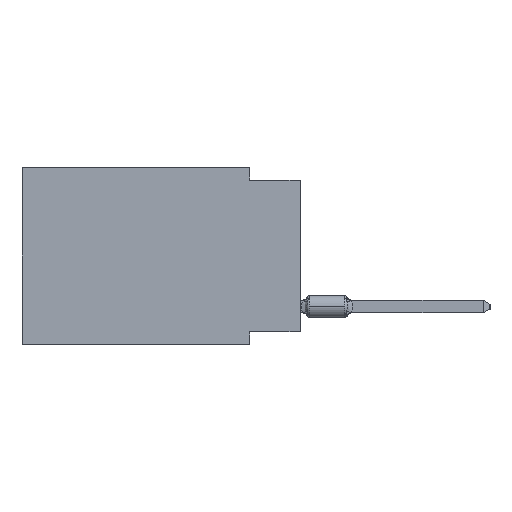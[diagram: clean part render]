
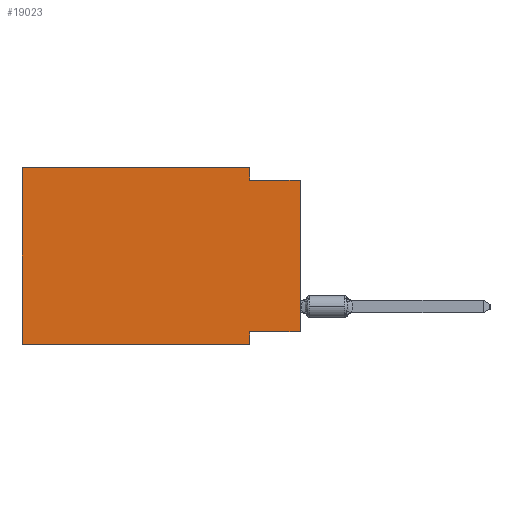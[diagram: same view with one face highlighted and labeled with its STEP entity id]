
A CAD part, left-side view. The second image highlights one B-rep face of the part: STEP entity #19023.
In plain terms, the highlighted planar face has unit normal (-1, 0, 0).
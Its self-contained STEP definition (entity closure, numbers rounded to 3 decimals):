
#446 = LINE ( 'NONE', #13883, #42540 ) ;
#493 = VERTEX_POINT ( 'NONE', #34666 ) ;
#707 = VECTOR ( 'NONE', #30451, 1000. ) ;
#3719 = EDGE_CURVE ( 'NONE', #34010, #19646, #17019, .T. ) ;
#3943 = EDGE_CURVE ( 'NONE', #493, #41448, #23555, .T. ) ;
#4570 = LINE ( 'NONE', #11163, #5122 ) ;
#5122 = VECTOR ( 'NONE', #38279, 1000. ) ;
#7611 = CARTESIAN_POINT ( 'NONE',  ( 0., 2.54, -8.89 ) ) ;
#7766 = DIRECTION ( 'NONE',  ( 1., 0., 0. ) ) ;
#9328 = AXIS2_PLACEMENT_3D ( 'NONE', #35085, #7766, #20788 ) ;
#9419 = DIRECTION ( 'NONE',  ( 0., 0., 1. ) ) ;
#10802 = EDGE_CURVE ( 'NONE', #40363, #19696, #25728, .T. ) ;
#11163 = CARTESIAN_POINT ( 'NONE',  ( 0., 0., -0.635 ) ) ;
#11625 = ORIENTED_EDGE ( 'NONE', *, *, #13095, .F. ) ;
#13095 = EDGE_CURVE ( 'NONE', #16051, #25319, #21455, .T. ) ;
#13883 = CARTESIAN_POINT ( 'NONE',  ( 0., 0., -8.255 ) ) ;
#14962 = EDGE_CURVE ( 'NONE', #40363, #16051, #446, .T. ) ;
#15193 = ORIENTED_EDGE ( 'NONE', *, *, #14962, .F. ) ;
#16023 = ORIENTED_EDGE ( 'NONE', *, *, #22219, .F. ) ;
#16051 = VERTEX_POINT ( 'NONE', #30290 ) ;
#17019 = LINE ( 'NONE', #26502, #707 ) ;
#17231 = VECTOR ( 'NONE', #34895, 1000. ) ;
#17383 = CARTESIAN_POINT ( 'NONE',  ( 0., 13.97, 0. ) ) ;
#17529 = LINE ( 'NONE', #40897, #19198 ) ;
#17922 = PLANE ( 'NONE',  #9328 ) ;
#18116 = VECTOR ( 'NONE', #9419, 1000. ) ;
#19023 = ADVANCED_FACE ( 'NONE', ( #30897 ), #17922, .F. ) ;
#19198 = VECTOR ( 'NONE', #27879, 1000. ) ;
#19646 = VERTEX_POINT ( 'NONE', #20184 ) ;
#19696 = VERTEX_POINT ( 'NONE', #34489 ) ;
#20017 = DIRECTION ( 'NONE',  ( 0., -1., 0. ) ) ;
#20184 = CARTESIAN_POINT ( 'NONE',  ( 0., 2.54, -0.635 ) ) ;
#20716 = DIRECTION ( 'NONE',  ( 0., 1., 0. ) ) ;
#20788 = DIRECTION ( 'NONE',  ( 0., 0., -1. ) ) ;
#21455 = LINE ( 'NONE', #24981, #17231 ) ;
#21679 = ORIENTED_EDGE ( 'NONE', *, *, #3719, .F. ) ;
#22219 = EDGE_CURVE ( 'NONE', #19646, #19696, #4570, .T. ) ;
#22516 = ORIENTED_EDGE ( 'NONE', *, *, #10802, .T. ) ;
#23314 = CARTESIAN_POINT ( 'NONE',  ( 0., 13.97, 0. ) ) ;
#23328 = DIRECTION ( 'NONE',  ( 0., 0., 1. ) ) ;
#23555 = LINE ( 'NONE', #17383, #42239 ) ;
#23612 = EDGE_CURVE ( 'NONE', #41448, #34010, #39651, .T. ) ;
#24981 = CARTESIAN_POINT ( 'NONE',  ( 0., 2.54, -8.89 ) ) ;
#25265 = EDGE_CURVE ( 'NONE', #493, #25319, #17529, .T. ) ;
#25319 = VERTEX_POINT ( 'NONE', #7611 ) ;
#25552 = VECTOR ( 'NONE', #20017, 1000. ) ;
#25728 = LINE ( 'NONE', #35850, #18116 ) ;
#26502 = CARTESIAN_POINT ( 'NONE',  ( 0., 2.54, 0. ) ) ;
#27879 = DIRECTION ( 'NONE',  ( 0., -1., 0. ) ) ;
#29566 = ORIENTED_EDGE ( 'NONE', *, *, #23612, .F. ) ;
#30290 = CARTESIAN_POINT ( 'NONE',  ( 0., 2.54, -8.255 ) ) ;
#30451 = DIRECTION ( 'NONE',  ( 0., 0., -1. ) ) ;
#30897 = FACE_OUTER_BOUND ( 'NONE', #34686, .T. ) ;
#31144 = CARTESIAN_POINT ( 'NONE',  ( 0., 2.54, 0. ) ) ;
#32423 = CARTESIAN_POINT ( 'NONE',  ( 0., 0., -8.255 ) ) ;
#34010 = VERTEX_POINT ( 'NONE', #31144 ) ;
#34489 = CARTESIAN_POINT ( 'NONE',  ( 0., 0., -0.635 ) ) ;
#34666 = CARTESIAN_POINT ( 'NONE',  ( 0., 13.97, -8.89 ) ) ;
#34686 = EDGE_LOOP ( 'NONE', ( #22516, #16023, #21679, #29566, #36831, #40676, #11625, #15193 ) ) ;
#34895 = DIRECTION ( 'NONE',  ( 0., 0., -1. ) ) ;
#35085 = CARTESIAN_POINT ( 'NONE',  ( 0., 13.97, 0. ) ) ;
#35850 = CARTESIAN_POINT ( 'NONE',  ( 0., 0., 0. ) ) ;
#36831 = ORIENTED_EDGE ( 'NONE', *, *, #3943, .F. ) ;
#37610 = CARTESIAN_POINT ( 'NONE',  ( 0., 13.97, 0. ) ) ;
#38279 = DIRECTION ( 'NONE',  ( 0., -1., 0. ) ) ;
#39651 = LINE ( 'NONE', #23314, #25552 ) ;
#40363 = VERTEX_POINT ( 'NONE', #32423 ) ;
#40676 = ORIENTED_EDGE ( 'NONE', *, *, #25265, .T. ) ;
#40897 = CARTESIAN_POINT ( 'NONE',  ( 0., 13.97, -8.89 ) ) ;
#41448 = VERTEX_POINT ( 'NONE', #37610 ) ;
#42239 = VECTOR ( 'NONE', #23328, 1000. ) ;
#42540 = VECTOR ( 'NONE', #20716, 1000. ) ;
